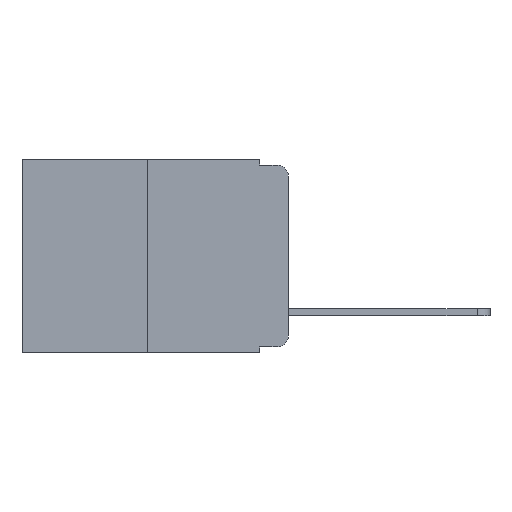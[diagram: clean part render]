
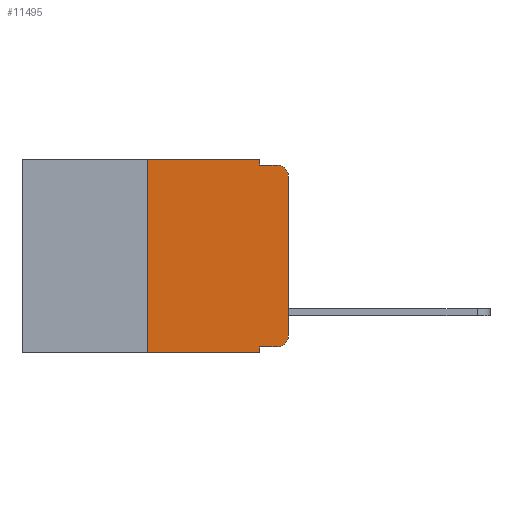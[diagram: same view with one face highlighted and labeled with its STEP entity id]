
A CAD part, left-side view. The second image highlights one B-rep face of the part: STEP entity #11495.
In plain terms, the highlighted planar face has unit normal (-1, 0, 0).
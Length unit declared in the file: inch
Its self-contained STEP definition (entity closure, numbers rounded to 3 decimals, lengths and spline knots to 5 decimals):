
#71 = CARTESIAN_POINT ( 'NONE',  ( 0., 0.02, -0.333 ) ) ;
#115 = EDGE_CURVE ( 'NONE', #526, #12552, #2658, .T. ) ;
#235 = CARTESIAN_POINT ( 'NONE',  ( 0., 0.051, 0. ) ) ;
#526 = VERTEX_POINT ( 'NONE', #13797 ) ;
#691 = EDGE_CURVE ( 'NONE', #9465, #5076, #2845, .T. ) ;
#719 = CARTESIAN_POINT ( 'NONE',  ( 0., 0.051, -0.01 ) ) ;
#1192 = CARTESIAN_POINT ( 'NONE',  ( 0., 0.473, -0.343 ) ) ;
#1321 = ORIENTED_EDGE ( 'NONE', *, *, #1389, .T. ) ;
#1389 = EDGE_CURVE ( 'NONE', #526, #13093, #2847, .T. ) ;
#1723 = ORIENTED_EDGE ( 'NONE', *, *, #3665, .T. ) ;
#1877 = DIRECTION ( 'NONE',  ( 0., -1., 0. ) ) ;
#2133 = VECTOR ( 'NONE', #4674, 39.37008 ) ;
#2541 = VERTEX_POINT ( 'NONE', #17210 ) ;
#2658 = LINE ( 'NONE', #11056, #16488 ) ;
#2706 = VECTOR ( 'NONE', #1877, 39.37008 ) ;
#2710 = VECTOR ( 'NONE', #9261, 39.37008 ) ;
#2845 = LINE ( 'NONE', #10500, #16672 ) ;
#2847 = LINE ( 'NONE', #11065, #16674 ) ;
#2937 = DIRECTION ( 'NONE',  ( 1., 0., 0. ) ) ;
#3281 = CARTESIAN_POINT ( 'NONE',  ( 0., 0.473, 0. ) ) ;
#3292 = AXIS2_PLACEMENT_3D ( 'NONE', #16274, #2937, #12312 ) ;
#3549 = LINE ( 'NONE', #3281, #2706 ) ;
#3665 = EDGE_CURVE ( 'NONE', #17286, #2541, #7792, .T. ) ;
#3763 = EDGE_CURVE ( 'NONE', #10431, #12984, #6546, .T. ) ;
#4234 = PLANE ( 'NONE',  #3292 ) ;
#4385 = CARTESIAN_POINT ( 'NONE',  ( 0., 0.25, -0.343 ) ) ;
#4523 = DIRECTION ( 'NONE',  ( 0., 0., -1. ) ) ;
#4674 = DIRECTION ( 'NONE',  ( 0., 0., 1. ) ) ;
#5038 = VECTOR ( 'NONE', #14174, 39.37008 ) ;
#5076 = VERTEX_POINT ( 'NONE', #9765 ) ;
#5321 = CARTESIAN_POINT ( 'NONE',  ( 0., 0.051, -0.343 ) ) ;
#5643 = CARTESIAN_POINT ( 'NONE',  ( 0., 0.02, -0.313 ) ) ;
#5732 = LINE ( 'NONE', #14022, #2133 ) ;
#6207 = EDGE_LOOP ( 'NONE', ( #10337, #1723, #10547, #16188, #10766, #16409, #10986, #9540, #1321, #17244 ) ) ;
#6546 = LINE ( 'NONE', #15537, #16791 ) ;
#6947 = EDGE_CURVE ( 'NONE', #12984, #9465, #3549, .T. ) ;
#6987 = DIRECTION ( 'NONE',  ( 0., 0., -1. ) ) ;
#7004 = DIRECTION ( 'NONE',  ( 0., 0., -1. ) ) ;
#7035 = DIRECTION ( 'NONE',  ( -1., 0., 0. ) ) ;
#7041 = EDGE_CURVE ( 'NONE', #5076, #2541, #16102, .T. ) ;
#7053 = CARTESIAN_POINT ( 'NONE',  ( 0., 0.02, -0.03 ) ) ;
#7792 = CIRCLE ( 'NONE', #14273, 0.02 ) ;
#7904 = VERTEX_POINT ( 'NONE', #16834 ) ;
#8857 = DIRECTION ( 'NONE',  ( 0., 0., 1. ) ) ;
#9261 = DIRECTION ( 'NONE',  ( 0., -1., 0. ) ) ;
#9342 = CARTESIAN_POINT ( 'NONE',  ( 0., 0.25, 0. ) ) ;
#9376 = AXIS2_PLACEMENT_3D ( 'NONE', #5643, #14986, #6987 ) ;
#9465 = VERTEX_POINT ( 'NONE', #235 ) ;
#9540 = ORIENTED_EDGE ( 'NONE', *, *, #115, .F. ) ;
#9765 = CARTESIAN_POINT ( 'NONE',  ( 0., 0.051, -0.01 ) ) ;
#10337 = ORIENTED_EDGE ( 'NONE', *, *, #16218, .T. ) ;
#10431 = VERTEX_POINT ( 'NONE', #4385 ) ;
#10500 = CARTESIAN_POINT ( 'NONE',  ( 0., 0.051, 0. ) ) ;
#10547 = ORIENTED_EDGE ( 'NONE', *, *, #7041, .F. ) ;
#10766 = ORIENTED_EDGE ( 'NONE', *, *, #6947, .F. ) ;
#10986 = ORIENTED_EDGE ( 'NONE', *, *, #11943, .T. ) ;
#11056 = CARTESIAN_POINT ( 'NONE',  ( 0., 0.051, 0. ) ) ;
#11065 = CARTESIAN_POINT ( 'NONE',  ( 0., 0.051, -0.333 ) ) ;
#11495 = ADVANCED_FACE ( 'NONE', ( #16552 ), #4234, .F. ) ;
#11943 = EDGE_CURVE ( 'NONE', #10431, #12552, #16948, .T. ) ;
#12290 = CARTESIAN_POINT ( 'NONE',  ( 0., 0., -0.03 ) ) ;
#12312 = DIRECTION ( 'NONE',  ( 0., 0., -1. ) ) ;
#12552 = VERTEX_POINT ( 'NONE', #5321 ) ;
#12984 = VERTEX_POINT ( 'NONE', #9342 ) ;
#13049 = DIRECTION ( 'NONE',  ( 0., -1., 0. ) ) ;
#13093 = VERTEX_POINT ( 'NONE', #71 ) ;
#13797 = CARTESIAN_POINT ( 'NONE',  ( 0., 0.051, -0.333 ) ) ;
#14022 = CARTESIAN_POINT ( 'NONE',  ( 0., 0., 0. ) ) ;
#14031 = DIRECTION ( 'NONE',  ( 0., 0., -1. ) ) ;
#14174 = DIRECTION ( 'NONE',  ( 0., -1., 0. ) ) ;
#14273 = AXIS2_PLACEMENT_3D ( 'NONE', #7053, #7035, #7004 ) ;
#14986 = DIRECTION ( 'NONE',  ( -1., 0., 0. ) ) ;
#15534 = EDGE_CURVE ( 'NONE', #13093, #7904, #16801, .T. ) ;
#15537 = CARTESIAN_POINT ( 'NONE',  ( 0., 0.25, 0. ) ) ;
#16102 = LINE ( 'NONE', #719, #5038 ) ;
#16188 = ORIENTED_EDGE ( 'NONE', *, *, #691, .F. ) ;
#16218 = EDGE_CURVE ( 'NONE', #7904, #17286, #5732, .T. ) ;
#16274 = CARTESIAN_POINT ( 'NONE',  ( 0., 0.473, 0. ) ) ;
#16409 = ORIENTED_EDGE ( 'NONE', *, *, #3763, .F. ) ;
#16488 = VECTOR ( 'NONE', #14031, 39.37008 ) ;
#16552 = FACE_OUTER_BOUND ( 'NONE', #6207, .T. ) ;
#16672 = VECTOR ( 'NONE', #4523, 39.37008 ) ;
#16674 = VECTOR ( 'NONE', #13049, 39.37008 ) ;
#16791 = VECTOR ( 'NONE', #8857, 39.37008 ) ;
#16801 = CIRCLE ( 'NONE', #9376, 0.02 ) ;
#16834 = CARTESIAN_POINT ( 'NONE',  ( 0., 0., -0.313 ) ) ;
#16948 = LINE ( 'NONE', #1192, #2710 ) ;
#17210 = CARTESIAN_POINT ( 'NONE',  ( 0., 0.02, -0.01 ) ) ;
#17244 = ORIENTED_EDGE ( 'NONE', *, *, #15534, .T. ) ;
#17286 = VERTEX_POINT ( 'NONE', #12290 ) ;
